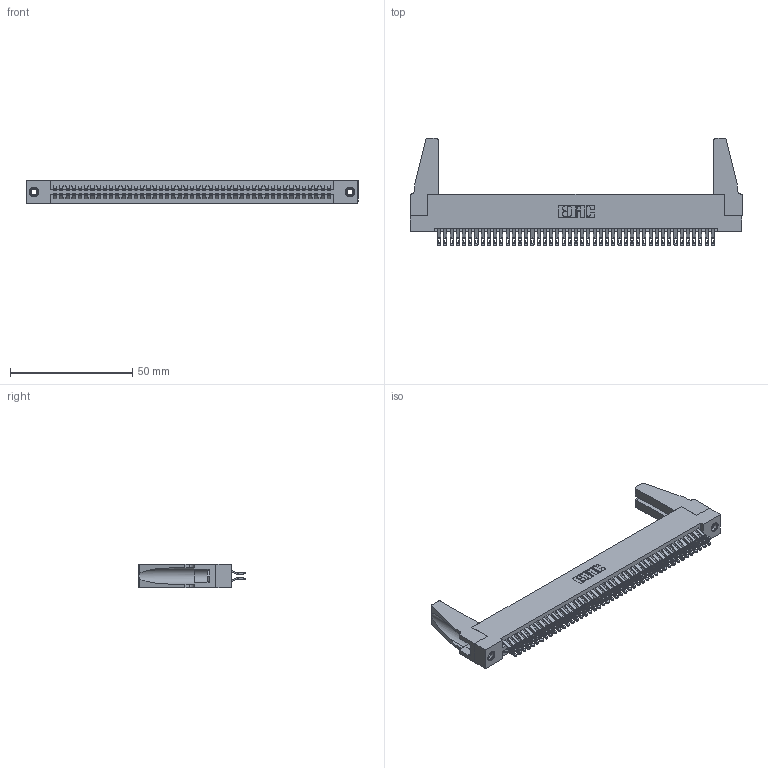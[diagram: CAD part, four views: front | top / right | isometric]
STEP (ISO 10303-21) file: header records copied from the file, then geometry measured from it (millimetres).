
FILE_DESCRIPTION (( 'STEP AP203' ), '1' );
FILE_NAME ('395-090-555-288.STEP', '2019-10-25T17:21:27', ( '' ), ( '' ), 'SwSTEP 2.0', 'SolidWorks 2016', '' );
FILE_SCHEMA (( 'CONFIG_CONTROL_DESIGN' ));
Length unit declared in the file: inch
Products named in the file (5): 345-250-001_345-250-001-102; 345-220-078_345-220-088; 395-090-555-288; 345 Part_Flush Mounting Lugs - 0.156 Dia-TH; 345-292-001_555 Tail
Assembly tree (95 placements, depth 2):
  395-090-555-288
    345 Part_Flush Mounting Lugs - 0.156 Dia-TH
    345-292-001_555 Tail  x90
    345-250-001_345-250-001-102  x2
    345-220-078_345-220-088  x2
Bounding box: 135.53 x 43.99 x 9.4 mm (x, y, z)
Volume: 16707.3 mm3; surface area: 23976.7 mm2
Topology: 95 solids, 95 shells, 5290 faces, 16585 edges, 11046 vertices
Faces by surface type: plane 2942, cylinder 2332, cone 12, torus 4
Entity records: 37378 total; most frequent: CARTESIAN_POINT 6292, ORIENTED_EDGE 6156, DIRECTION 5518, EDGE_CURVE 3078, VECTOR 2704, LINE 2704, VERTEX_POINT 2046, AXIS2_PLACEMENT_3D 1407
